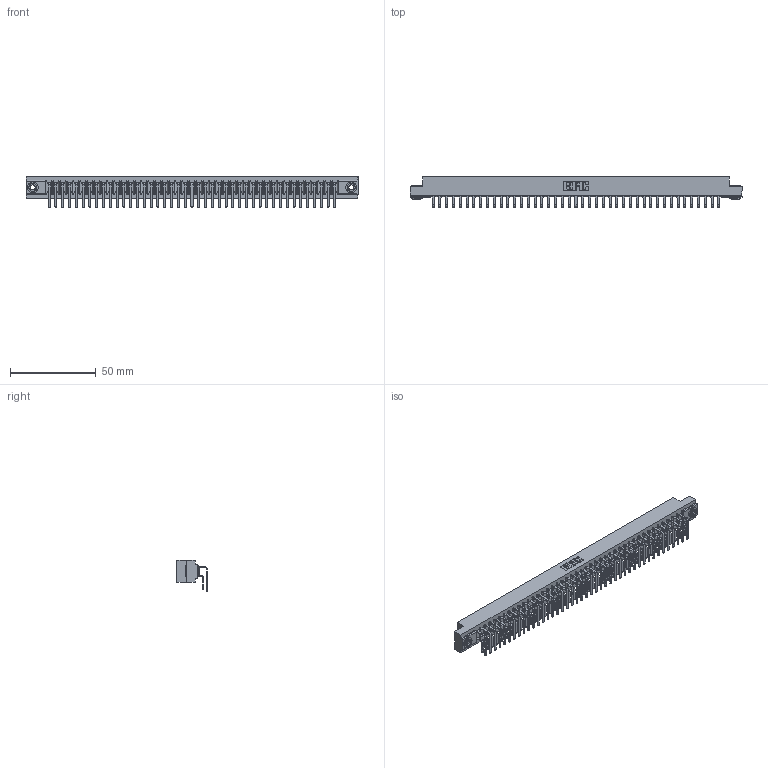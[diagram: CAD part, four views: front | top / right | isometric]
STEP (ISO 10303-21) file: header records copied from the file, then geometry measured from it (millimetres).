
FILE_DESCRIPTION (( 'STEP AP203' ), '1' );
FILE_NAME ('357-086-559-203.STEP', '2018-08-13T02:54:31', ( '' ), ( '' ), 'SwSTEP 2.0', 'SolidWorks 2016', '' );
FILE_SCHEMA (( 'CONFIG_CONTROL_DESIGN' ));
Length unit declared in the file: inch
Products named in the file (5): 357-086-559-203; 345-250-002_345-250-002-102; 307 Part_.156 Dia Mounting Holes; 307-290-001_558 559 - 1 (Single); 307-290-001_559 - 2 (Single)
Assembly tree (89 placements, depth 2):
  357-086-559-203
    307 Part_.156 Dia Mounting Holes
    307-290-001_558 559 - 1 (Single)  x43
    307-290-001_559 - 2 (Single)  x43
    345-250-002_345-250-002-102  x2
Bounding box: 193.4 x 17.69 x 18.07 mm (x, y, z)
Volume: 20955 mm3; surface area: 28131.4 mm2
Topology: 89 solids, 89 shells, 4514 faces, 12647 edges, 8194 vertices
Faces by surface type: plane 2932, cylinder 1486, sphere 88, cone 8
Entity records: 40628 total; most frequent: CARTESIAN_POINT 6630, ORIENTED_EDGE 6562, DIRECTION 6507, EDGE_CURVE 3281, VECTOR 2509, LINE 2509, VERTEX_POINT 2122, AXIS2_PLACEMENT_3D 1999
